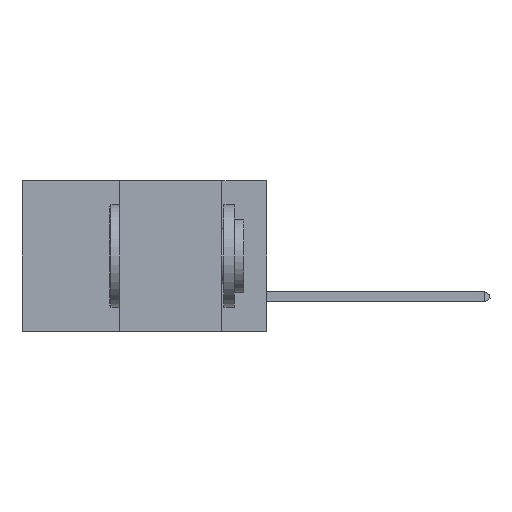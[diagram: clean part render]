
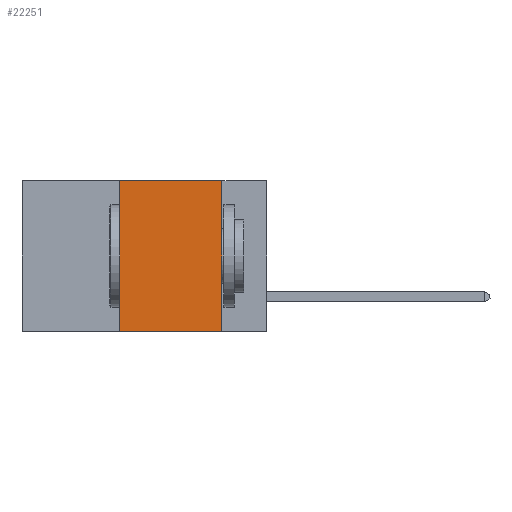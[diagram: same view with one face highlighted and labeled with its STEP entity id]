
A CAD part, left-side view. The second image highlights one B-rep face of the part: STEP entity #22251.
In plain terms, the highlighted planar face has unit normal (-1, 0, 0).
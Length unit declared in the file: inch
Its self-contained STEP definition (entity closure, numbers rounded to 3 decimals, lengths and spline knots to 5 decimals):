
#1413 = ORIENTED_EDGE ( 'NONE', *, *, #26691, .T. ) ;
#1839 = CARTESIAN_POINT ( 'NONE',  ( 0., 0.6, 0. ) ) ;
#2807 = LINE ( 'NONE', #15827, #17482 ) ;
#4253 = CARTESIAN_POINT ( 'NONE',  ( 0., 0.6, 0. ) ) ;
#6233 = VERTEX_POINT ( 'NONE', #7508 ) ;
#7008 = DIRECTION ( 'NONE',  ( 0., 0., 1. ) ) ;
#7165 = CARTESIAN_POINT ( 'NONE',  ( 0., 0.36, 0. ) ) ;
#7508 = CARTESIAN_POINT ( 'NONE',  ( 0., 0.36, -0.37 ) ) ;
#8362 = ORIENTED_EDGE ( 'NONE', *, *, #17352, .F. ) ;
#9326 = EDGE_LOOP ( 'NONE', ( #26624, #28327, #8362, #1413 ) ) ;
#9529 = VERTEX_POINT ( 'NONE', #7165 ) ;
#10187 = DIRECTION ( 'NONE',  ( 1., 0., 0. ) ) ;
#10357 = VERTEX_POINT ( 'NONE', #25173 ) ;
#11283 = CARTESIAN_POINT ( 'NONE',  ( 0., 0.6, -0.37 ) ) ;
#14413 = EDGE_CURVE ( 'NONE', #10357, #18921, #30210, .T. ) ;
#15068 = AXIS2_PLACEMENT_3D ( 'NONE', #4253, #10187, #29919 ) ;
#15383 = VECTOR ( 'NONE', #28575, 39.37008 ) ;
#15450 = EDGE_CURVE ( 'NONE', #9529, #10357, #23802, .T. ) ;
#15630 = LINE ( 'NONE', #11283, #21435 ) ;
#15827 = CARTESIAN_POINT ( 'NONE',  ( 0., 0.36, 0. ) ) ;
#16906 = FACE_OUTER_BOUND ( 'NONE', #9326, .T. ) ;
#17352 = EDGE_CURVE ( 'NONE', #6233, #9529, #2807, .T. ) ;
#17482 = VECTOR ( 'NONE', #7008, 39.37008 ) ;
#18838 = PLANE ( 'NONE',  #15068 ) ;
#18921 = VERTEX_POINT ( 'NONE', #33088 ) ;
#19370 = DIRECTION ( 'NONE',  ( 0., -1., 0. ) ) ;
#21435 = VECTOR ( 'NONE', #28288, 39.37008 ) ;
#22251 = ADVANCED_FACE ( 'NONE', ( #16906 ), #18838, .F. ) ;
#23802 = LINE ( 'NONE', #1839, #30181 ) ;
#25173 = CARTESIAN_POINT ( 'NONE',  ( 0., 0.11, 0. ) ) ;
#25849 = CARTESIAN_POINT ( 'NONE',  ( 0., 0.11, 0. ) ) ;
#26624 = ORIENTED_EDGE ( 'NONE', *, *, #14413, .F. ) ;
#26691 = EDGE_CURVE ( 'NONE', #6233, #18921, #15630, .T. ) ;
#28288 = DIRECTION ( 'NONE',  ( 0., -1., 0. ) ) ;
#28327 = ORIENTED_EDGE ( 'NONE', *, *, #15450, .F. ) ;
#28575 = DIRECTION ( 'NONE',  ( 0., 0., -1. ) ) ;
#29919 = DIRECTION ( 'NONE',  ( 0., 0., -1. ) ) ;
#30181 = VECTOR ( 'NONE', #19370, 39.37008 ) ;
#30210 = LINE ( 'NONE', #25849, #15383 ) ;
#33088 = CARTESIAN_POINT ( 'NONE',  ( 0., 0.11, -0.37 ) ) ;
